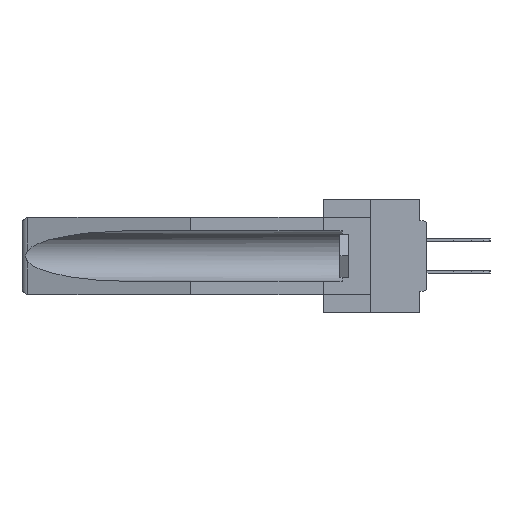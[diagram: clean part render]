
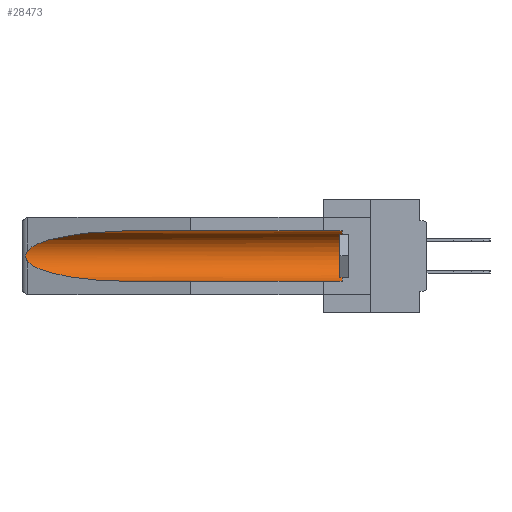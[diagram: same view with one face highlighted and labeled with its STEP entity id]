
A CAD part, left-side view. The second image highlights one B-rep face of the part: STEP entity #28473.
In plain terms, the highlighted cylindrical face has radius 2.857 mm (diameter 5.715 mm), a partial arc.
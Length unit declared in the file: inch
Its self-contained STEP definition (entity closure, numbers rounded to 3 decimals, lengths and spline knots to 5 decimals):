
#983 = CARTESIAN_POINT ( 'NONE',  ( 0.21114, 1.30732, -0.059 ) ) ;
#1227 = DIRECTION ( 'NONE',  ( 0., -1., 0. ) ) ;
#1440 = ORIENTED_EDGE ( 'NONE', *, *, #20930, .T. ) ;
#1506 = ORIENTED_EDGE ( 'NONE', *, *, #45249, .T. ) ;
#3085 = ORIENTED_EDGE ( 'NONE', *, *, #5039, .F. ) ;
#3262 = VERTEX_POINT ( 'NONE', #23086 ) ;
#4933 = VECTOR ( 'NONE', #41166, 39.37008 ) ;
#5039 = EDGE_CURVE ( 'NONE', #12245, #3262, #29329, .T. ) ;
#5255 = DIRECTION ( 'NONE',  ( 0., 0., 1. ) ) ;
#6105 = VECTOR ( 'NONE', #36867, 39.37008 ) ;
#9277 = CIRCLE ( 'NONE', #19702, 0.1125 ) ;
#9692 = CARTESIAN_POINT ( 'NONE',  ( 0.26654, 1.53092, -0.15636 ) ) ;
#11891 = CARTESIAN_POINT ( 'NONE',  ( 0.155, 1.07973, -0.284 ) ) ;
#12159 = CARTESIAN_POINT ( 'NONE',  ( 0.25451, 1.48313, -0.09465 ) ) ;
#12245 = VERTEX_POINT ( 'NONE', #34045 ) ;
#12725 = CARTESIAN_POINT ( 'NONE',  ( 0.155, 1.07973, -0.059 ) ) ;
#12982 = EDGE_CURVE ( 'NONE', #12245, #14265, #9277, .T. ) ;
#14265 = VERTEX_POINT ( 'NONE', #24449 ) ;
#14395 =( BOUNDED_CURVE ( )  B_SPLINE_CURVE ( 3, ( #15394, #983, #12159, #40261 ),
 .UNSPECIFIED., .F., .F. ) 
 B_SPLINE_CURVE_WITH_KNOTS ( ( 4, 4 ),
 ( 4.71239, 6.08839 ),
 .UNSPECIFIED. ) 
 CURVE ( )  GEOMETRIC_REPRESENTATION_ITEM ( )  RATIONAL_B_SPLINE_CURVE ( ( 1., 0.848, 0.848, 1. ) ) 
 REPRESENTATION_ITEM ( '' )  );
#15394 = CARTESIAN_POINT ( 'NONE',  ( 0.155, 1.07973, -0.059 ) ) ;
#16520 = CARTESIAN_POINT ( 'NONE',  ( 0.26597, 1.52961, -0.15275 ) ) ;
#16673 = LINE ( 'NONE', #26415, #6105 ) ;
#17840 = EDGE_CURVE ( 'NONE', #38911, #3262, #26071, .T. ) ;
#18394 = CARTESIAN_POINT ( 'NONE',  ( 0.155, -0.30754, -0.1715 ) ) ;
#18871 = CARTESIAN_POINT ( 'NONE',  ( 0.25451, 1.48313, -0.24835 ) ) ;
#19702 = AXIS2_PLACEMENT_3D ( 'NONE', #36792, #1227, #5255 ) ;
#19794 = CARTESIAN_POINT ( 'NONE',  ( 0.26597, 1.5296, -0.19026 ) ) ;
#20411 = CARTESIAN_POINT ( 'NONE',  ( 0.2673, 1.53269, -0.17917 ) ) ;
#20930 = EDGE_CURVE ( 'NONE', #14265, #35346, #16673, .T. ) ;
#23086 = CARTESIAN_POINT ( 'NONE',  ( 0.155, 1.07973, -0.284 ) ) ;
#23318 = CYLINDRICAL_SURFACE ( 'NONE', #42308, 0.1125 ) ;
#23523 = CARTESIAN_POINT ( 'NONE',  ( 0.26655, 1.53094, -0.18657 ) ) ;
#23836 = CARTESIAN_POINT ( 'NONE',  ( 0.2675, 1.53308, -0.16763 ) ) ;
#23993 = CARTESIAN_POINT ( 'NONE',  ( 0.26537, 1.52718, -0.19328 ) ) ;
#24449 = CARTESIAN_POINT ( 'NONE',  ( 0.155, 0.126, -0.059 ) ) ;
#25981 = DIRECTION ( 'NONE',  ( 0., 1., 0. ) ) ;
#26071 =( BOUNDED_CURVE ( )  B_SPLINE_CURVE ( 3, ( #40145, #18871, #39843, #11891 ),
 .UNSPECIFIED., .F., .F. ) 
 B_SPLINE_CURVE_WITH_KNOTS ( ( 4, 4 ),
 ( 0.1948, 1.5708 ),
 .UNSPECIFIED. ) 
 CURVE ( )  GEOMETRIC_REPRESENTATION_ITEM ( )  RATIONAL_B_SPLINE_CURVE ( ( 1., 0.848, 0.848, 1. ) ) 
 REPRESENTATION_ITEM ( '' )  );
#26415 = CARTESIAN_POINT ( 'NONE',  ( 0.155, -0.30754, -0.059 ) ) ;
#26634 = FACE_OUTER_BOUND ( 'NONE', #28344, .T. ) ;
#26904 = B_SPLINE_CURVE_WITH_KNOTS ( 'NONE', 3,
 ( #30349, #16520, #9692, #41693, #23836, #41073, #20411, #23523, #19794, #23993 ),
 .UNSPECIFIED., .F., .F.,
 ( 4, 2, 2, 2, 4 ),
 ( 0., 0.00029, 0.00058, 0.00087, 0.00117 ),
 .UNSPECIFIED. ) ;
#28344 = EDGE_LOOP ( 'NONE', ( #1506, #38318, #34183, #3085, #31261, #1440 ) ) ;
#28473 = ADVANCED_FACE ( 'NONE', ( #26634 ), #23318, .F. ) ;
#29329 = LINE ( 'NONE', #44413, #4933 ) ;
#30349 = CARTESIAN_POINT ( 'NONE',  ( 0.26537, 1.52718, -0.14972 ) ) ;
#30478 = CARTESIAN_POINT ( 'NONE',  ( 0.26537, 1.52718, -0.19328 ) ) ;
#31261 = ORIENTED_EDGE ( 'NONE', *, *, #12982, .T. ) ;
#34045 = CARTESIAN_POINT ( 'NONE',  ( 0.155, 0.126, -0.284 ) ) ;
#34183 = ORIENTED_EDGE ( 'NONE', *, *, #17840, .T. ) ;
#34381 = CARTESIAN_POINT ( 'NONE',  ( 0.26537, 1.52718, -0.14972 ) ) ;
#35346 = VERTEX_POINT ( 'NONE', #12725 ) ;
#36792 = CARTESIAN_POINT ( 'NONE',  ( 0.155, 0.126, -0.1715 ) ) ;
#36867 = DIRECTION ( 'NONE',  ( 0., 1., 0. ) ) ;
#37340 = DIRECTION ( 'NONE',  ( 0., 0., 1. ) ) ;
#38318 = ORIENTED_EDGE ( 'NONE', *, *, #44176, .T. ) ;
#38911 = VERTEX_POINT ( 'NONE', #30478 ) ;
#39843 = CARTESIAN_POINT ( 'NONE',  ( 0.21114, 1.30732, -0.284 ) ) ;
#40145 = CARTESIAN_POINT ( 'NONE',  ( 0.26537, 1.52718, -0.19328 ) ) ;
#40261 = CARTESIAN_POINT ( 'NONE',  ( 0.26537, 1.52718, -0.14972 ) ) ;
#41073 = CARTESIAN_POINT ( 'NONE',  ( 0.2675, 1.53308, -0.17534 ) ) ;
#41166 = DIRECTION ( 'NONE',  ( 0., 1., 0. ) ) ;
#41693 = CARTESIAN_POINT ( 'NONE',  ( 0.2673, 1.5327, -0.16383 ) ) ;
#42308 = AXIS2_PLACEMENT_3D ( 'NONE', #18394, #25981, #37340 ) ;
#42504 = VERTEX_POINT ( 'NONE', #34381 ) ;
#44176 = EDGE_CURVE ( 'NONE', #42504, #38911, #26904, .T. ) ;
#44413 = CARTESIAN_POINT ( 'NONE',  ( 0.155, -0.30754, -0.284 ) ) ;
#45249 = EDGE_CURVE ( 'NONE', #35346, #42504, #14395, .T. ) ;
